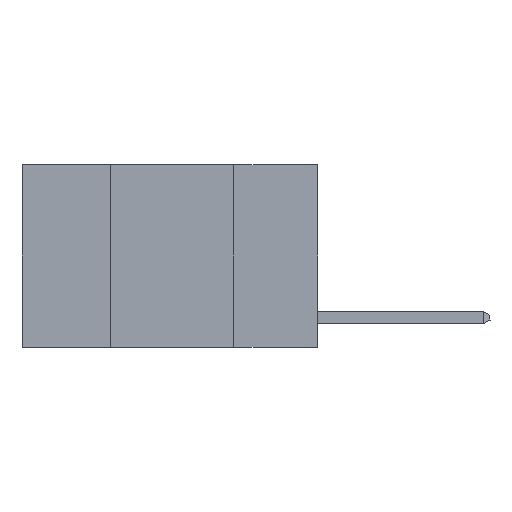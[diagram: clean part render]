
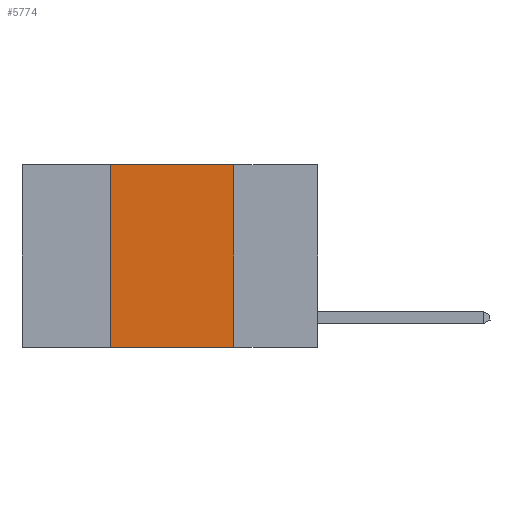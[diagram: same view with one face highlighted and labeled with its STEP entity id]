
A CAD part, left-side view. The second image highlights one B-rep face of the part: STEP entity #5774.
In plain terms, the highlighted planar face has unit normal (-1, 0, 0).
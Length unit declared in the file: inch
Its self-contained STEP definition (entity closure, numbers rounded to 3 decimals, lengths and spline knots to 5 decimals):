
#120 = EDGE_LOOP ( 'NONE', ( #1447, #7146, #7915, #1526 ) ) ;
#187 = DIRECTION ( 'NONE',  ( 1., 0., 0. ) ) ;
#582 = LINE ( 'NONE', #4223, #5734 ) ;
#1169 = VECTOR ( 'NONE', #4335, 39.37008 ) ;
#1447 = ORIENTED_EDGE ( 'NONE', *, *, #2916, .F. ) ;
#1526 = ORIENTED_EDGE ( 'NONE', *, *, #5088, .T. ) ;
#1742 = DIRECTION ( 'NONE',  ( 0., -1., 0. ) ) ;
#2156 = VECTOR ( 'NONE', #1742, 39.37008 ) ;
#2206 = VECTOR ( 'NONE', #5207, 39.37008 ) ;
#2439 = CARTESIAN_POINT ( 'NONE',  ( 0., 0.42, 0. ) ) ;
#2661 = AXIS2_PLACEMENT_3D ( 'NONE', #3415, #187, #4844 ) ;
#2916 = EDGE_CURVE ( 'NONE', #7033, #6882, #5804, .T. ) ;
#3095 = EDGE_CURVE ( 'NONE', #3529, #7033, #4684, .T. ) ;
#3415 = CARTESIAN_POINT ( 'NONE',  ( 0., 0.6, 0. ) ) ;
#3516 = CARTESIAN_POINT ( 'NONE',  ( 0., 0.17, -0.37 ) ) ;
#3529 = VERTEX_POINT ( 'NONE', #2439 ) ;
#3547 = FACE_OUTER_BOUND ( 'NONE', #120, .T. ) ;
#4223 = CARTESIAN_POINT ( 'NONE',  ( 0., 0.42, 0. ) ) ;
#4316 = CARTESIAN_POINT ( 'NONE',  ( 0., 0.6, 0. ) ) ;
#4335 = DIRECTION ( 'NONE',  ( 0., -1., 0. ) ) ;
#4576 = VERTEX_POINT ( 'NONE', #6986 ) ;
#4684 = LINE ( 'NONE', #4316, #1169 ) ;
#4844 = DIRECTION ( 'NONE',  ( 0., 0., -1. ) ) ;
#4928 = DIRECTION ( 'NONE',  ( 0., 0., 1. ) ) ;
#5088 = EDGE_CURVE ( 'NONE', #4576, #6882, #5746, .T. ) ;
#5207 = DIRECTION ( 'NONE',  ( 0., 0., -1. ) ) ;
#5285 = CARTESIAN_POINT ( 'NONE',  ( 0., 0.17, 0. ) ) ;
#5734 = VECTOR ( 'NONE', #4928, 39.37008 ) ;
#5746 = LINE ( 'NONE', #6496, #2156 ) ;
#5774 = ADVANCED_FACE ( 'NONE', ( #3547 ), #7573, .F. ) ;
#5804 = LINE ( 'NONE', #5285, #2206 ) ;
#6179 = EDGE_CURVE ( 'NONE', #4576, #3529, #582, .T. ) ;
#6469 = CARTESIAN_POINT ( 'NONE',  ( 0., 0.17, 0. ) ) ;
#6496 = CARTESIAN_POINT ( 'NONE',  ( 0., 0.6, -0.37 ) ) ;
#6882 = VERTEX_POINT ( 'NONE', #3516 ) ;
#6986 = CARTESIAN_POINT ( 'NONE',  ( 0., 0.42, -0.37 ) ) ;
#7033 = VERTEX_POINT ( 'NONE', #6469 ) ;
#7146 = ORIENTED_EDGE ( 'NONE', *, *, #3095, .F. ) ;
#7573 = PLANE ( 'NONE',  #2661 ) ;
#7915 = ORIENTED_EDGE ( 'NONE', *, *, #6179, .F. ) ;
